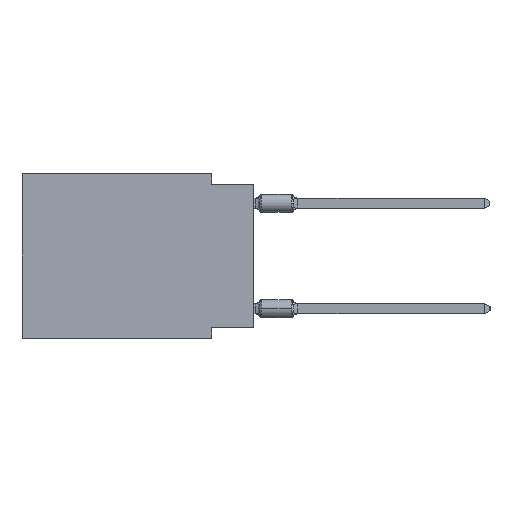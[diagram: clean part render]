
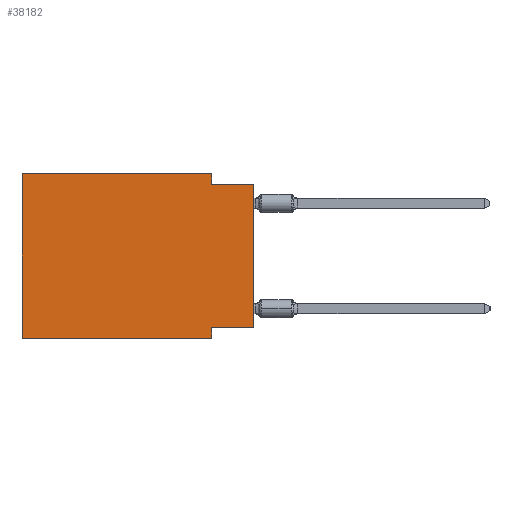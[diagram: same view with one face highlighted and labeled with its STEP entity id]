
A CAD part, left-side view. The second image highlights one B-rep face of the part: STEP entity #38182.
In plain terms, the highlighted planar face has unit normal (-1, 0, 0).
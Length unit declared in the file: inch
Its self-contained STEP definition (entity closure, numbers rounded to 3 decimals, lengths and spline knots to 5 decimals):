
#744 = CARTESIAN_POINT ( 'NONE',  ( 0., 0.55, 0. ) ) ;
#1722 = LINE ( 'NONE', #2187, #42626 ) ;
#2174 = ORIENTED_EDGE ( 'NONE', *, *, #40562, .F. ) ;
#2187 = CARTESIAN_POINT ( 'NONE',  ( 0., 0., 0. ) ) ;
#3796 = EDGE_LOOP ( 'NONE', ( #17773, #16084, #15072, #31418, #2174, #15915, #22674, #23378 ) ) ;
#3935 = CARTESIAN_POINT ( 'NONE',  ( 0., 0.55, 0. ) ) ;
#6821 = VECTOR ( 'NONE', #9835, 39.37008 ) ;
#7293 = CARTESIAN_POINT ( 'NONE',  ( 0., 0.1, -0.39 ) ) ;
#7823 = CARTESIAN_POINT ( 'NONE',  ( 0., 0.1, -0.365 ) ) ;
#8539 = VECTOR ( 'NONE', #35773, 39.37008 ) ;
#8643 = CARTESIAN_POINT ( 'NONE',  ( 0., 0.55, -0.39 ) ) ;
#9068 = LINE ( 'NONE', #45736, #16473 ) ;
#9659 = LINE ( 'NONE', #46812, #44872 ) ;
#9835 = DIRECTION ( 'NONE',  ( 0., 1., 0. ) ) ;
#11781 = CARTESIAN_POINT ( 'NONE',  ( 0., 0.1, 0. ) ) ;
#12450 = DIRECTION ( 'NONE',  ( 0., 0., -1. ) ) ;
#13455 = LINE ( 'NONE', #28279, #6821 ) ;
#13893 = EDGE_CURVE ( 'NONE', #28529, #28767, #17037, .T. ) ;
#15072 = ORIENTED_EDGE ( 'NONE', *, *, #38376, .F. ) ;
#15538 = LINE ( 'NONE', #744, #29251 ) ;
#15915 = ORIENTED_EDGE ( 'NONE', *, *, #26696, .T. ) ;
#16084 = ORIENTED_EDGE ( 'NONE', *, *, #39553, .F. ) ;
#16132 = CARTESIAN_POINT ( 'NONE',  ( 0., 0.55, -0.39 ) ) ;
#16473 = VECTOR ( 'NONE', #12450, 39.37008 ) ;
#16761 = AXIS2_PLACEMENT_3D ( 'NONE', #18879, #41256, #27128 ) ;
#17037 = LINE ( 'NONE', #17286, #8539 ) ;
#17286 = CARTESIAN_POINT ( 'NONE',  ( 0., 0.55, 0. ) ) ;
#17350 = EDGE_CURVE ( 'NONE', #43401, #20264, #9068, .T. ) ;
#17369 = CARTESIAN_POINT ( 'NONE',  ( 0., 0.1, 0. ) ) ;
#17773 = ORIENTED_EDGE ( 'NONE', *, *, #43640, .T. ) ;
#18879 = CARTESIAN_POINT ( 'NONE',  ( 0., 0.55, 0. ) ) ;
#20264 = VERTEX_POINT ( 'NONE', #7293 ) ;
#20767 = LINE ( 'NONE', #17369, #35419 ) ;
#22674 = ORIENTED_EDGE ( 'NONE', *, *, #17350, .F. ) ;
#23378 = ORIENTED_EDGE ( 'NONE', *, *, #41626, .F. ) ;
#23439 = DIRECTION ( 'NONE',  ( 0., -1., 0. ) ) ;
#24458 = DIRECTION ( 'NONE',  ( 0., -1., 0. ) ) ;
#24925 = DIRECTION ( 'NONE',  ( 0., 0., -1. ) ) ;
#26696 = EDGE_CURVE ( 'NONE', #39832, #20264, #30747, .T. ) ;
#27128 = DIRECTION ( 'NONE',  ( 0., 0., -1. ) ) ;
#28279 = CARTESIAN_POINT ( 'NONE',  ( 0., 0., -0.365 ) ) ;
#28529 = VERTEX_POINT ( 'NONE', #3935 ) ;
#28767 = VERTEX_POINT ( 'NONE', #11781 ) ;
#29251 = VECTOR ( 'NONE', #37914, 39.37008 ) ;
#29837 = FACE_OUTER_BOUND ( 'NONE', #3796, .T. ) ;
#30747 = LINE ( 'NONE', #8643, #31176 ) ;
#31176 = VECTOR ( 'NONE', #23439, 39.37008 ) ;
#31418 = ORIENTED_EDGE ( 'NONE', *, *, #13893, .F. ) ;
#33265 = VERTEX_POINT ( 'NONE', #41062 ) ;
#35419 = VECTOR ( 'NONE', #24925, 39.37008 ) ;
#35773 = DIRECTION ( 'NONE',  ( 0., -1., 0. ) ) ;
#37914 = DIRECTION ( 'NONE',  ( 0., 0., 1. ) ) ;
#38182 = ADVANCED_FACE ( 'NONE', ( #29837 ), #44664, .F. ) ;
#38376 = EDGE_CURVE ( 'NONE', #28767, #39600, #20767, .T. ) ;
#38802 = CARTESIAN_POINT ( 'NONE',  ( 0., 0.1, -0.025 ) ) ;
#39553 = EDGE_CURVE ( 'NONE', #39600, #33265, #9659, .T. ) ;
#39600 = VERTEX_POINT ( 'NONE', #38802 ) ;
#39832 = VERTEX_POINT ( 'NONE', #16132 ) ;
#40562 = EDGE_CURVE ( 'NONE', #39832, #28529, #15538, .T. ) ;
#41062 = CARTESIAN_POINT ( 'NONE',  ( 0., 0., -0.025 ) ) ;
#41256 = DIRECTION ( 'NONE',  ( 1., 0., 0. ) ) ;
#41626 = EDGE_CURVE ( 'NONE', #42703, #43401, #13455, .T. ) ;
#42626 = VECTOR ( 'NONE', #42997, 39.37008 ) ;
#42703 = VERTEX_POINT ( 'NONE', #46756 ) ;
#42997 = DIRECTION ( 'NONE',  ( 0., 0., 1. ) ) ;
#43401 = VERTEX_POINT ( 'NONE', #7823 ) ;
#43640 = EDGE_CURVE ( 'NONE', #42703, #33265, #1722, .T. ) ;
#44664 = PLANE ( 'NONE',  #16761 ) ;
#44872 = VECTOR ( 'NONE', #24458, 39.37008 ) ;
#45736 = CARTESIAN_POINT ( 'NONE',  ( 0., 0.1, -0.39 ) ) ;
#46756 = CARTESIAN_POINT ( 'NONE',  ( 0., 0., -0.365 ) ) ;
#46812 = CARTESIAN_POINT ( 'NONE',  ( 0., 0., -0.025 ) ) ;
